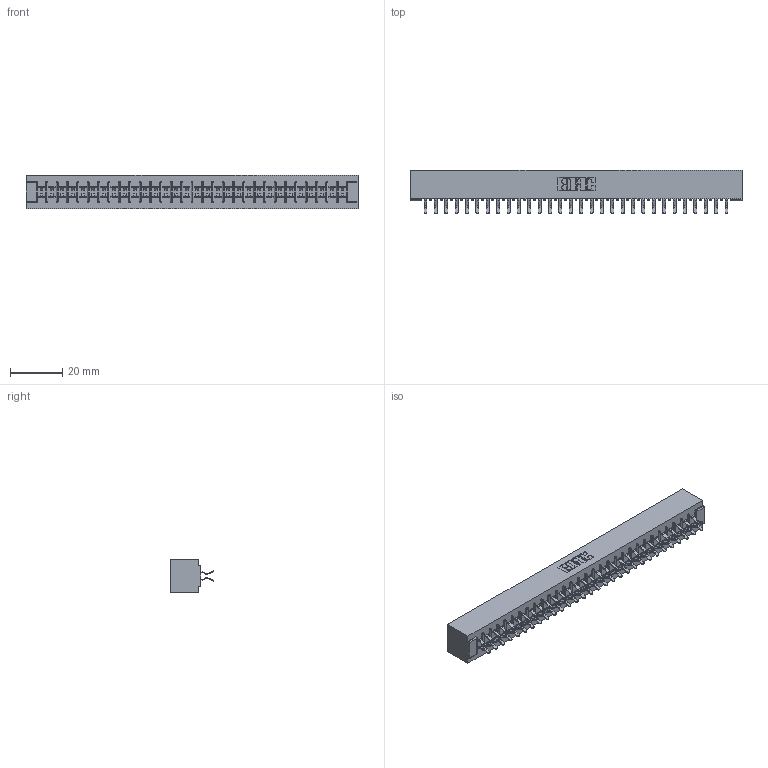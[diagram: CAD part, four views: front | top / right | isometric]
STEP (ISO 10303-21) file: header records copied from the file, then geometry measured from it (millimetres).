
FILE_DESCRIPTION (( 'STEP AP203' ), '1' );
FILE_NAME ('315-060-556-201.STEP', '2019-09-10T20:05:06', ( '' ), ( '' ), 'SwSTEP 2.0', 'SolidWorks 2016', '' );
FILE_SCHEMA (( 'CONFIG_CONTROL_DESIGN' ));
Length unit declared in the file: inch
Products named in the file (3): 305-290-001_556; 315-060-556-201; 305 Part_No Mounting
Assembly tree (61 placements, depth 2):
  315-060-556-201
    305 Part_No Mounting
    305-290-001_556  x60
Bounding box: 126.75 x 16.64 x 12.7 mm (x, y, z)
Volume: 13630.1 mm3; surface area: 17482.2 mm2
Topology: 61 solids, 61 shells, 3468 faces, 9982 edges, 6492 vertices
Faces by surface type: plane 1924, cylinder 1424, sphere 120
Entity records: 33887 total; most frequent: CARTESIAN_POINT 5608, ORIENTED_EDGE 5564, DIRECTION 5436, EDGE_CURVE 2782, LINE 2236, VECTOR 2236, VERTEX_POINT 1772, AXIS2_PLACEMENT_3D 1600
